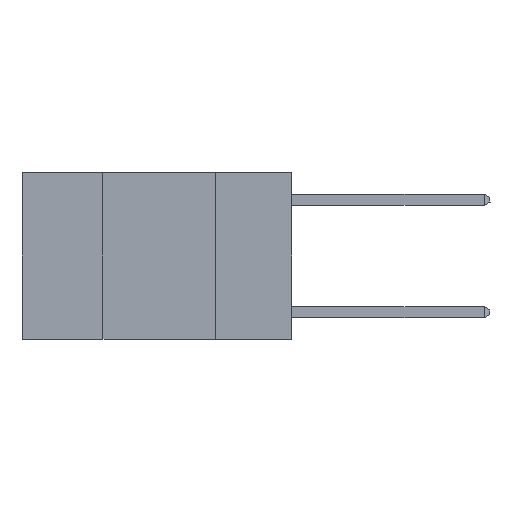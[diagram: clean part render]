
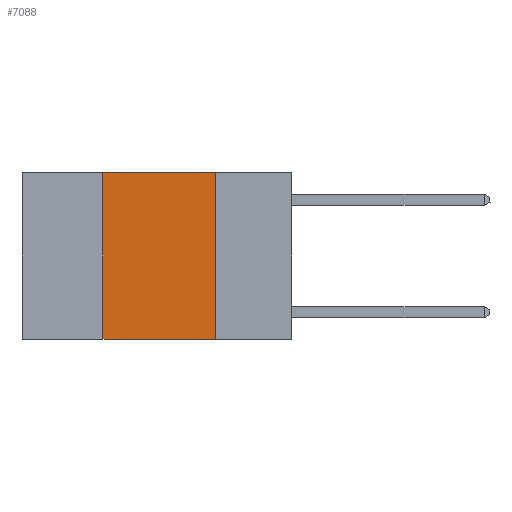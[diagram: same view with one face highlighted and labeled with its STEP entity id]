
A CAD part, left-side view. The second image highlights one B-rep face of the part: STEP entity #7088.
In plain terms, the highlighted planar face has unit normal (-1, 0, 0).
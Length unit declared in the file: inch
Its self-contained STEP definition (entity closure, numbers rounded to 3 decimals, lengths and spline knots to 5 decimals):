
#65 = CARTESIAN_POINT ( 'NONE',  ( 0., 0.6, 0. ) ) ;
#1277 = DIRECTION ( 'NONE',  ( 0., -1., 0. ) ) ;
#1431 = CARTESIAN_POINT ( 'NONE',  ( 0., 0.6, 0. ) ) ;
#1704 = LINE ( 'NONE', #65, #8877 ) ;
#2917 = DIRECTION ( 'NONE',  ( 0., 0., -1. ) ) ;
#5926 = CARTESIAN_POINT ( 'NONE',  ( 0., 0.42, -0.37 ) ) ;
#6629 = CARTESIAN_POINT ( 'NONE',  ( 0., 0.17, 0. ) ) ;
#7088 = ADVANCED_FACE ( 'NONE', ( #14624 ), #8603, .F. ) ;
#7216 = DIRECTION ( 'NONE',  ( 0., 0., 1. ) ) ;
#7532 = LINE ( 'NONE', #8627, #13760 ) ;
#8603 = PLANE ( 'NONE',  #8641 ) ;
#8627 = CARTESIAN_POINT ( 'NONE',  ( 0., 0.42, 0. ) ) ;
#8641 = AXIS2_PLACEMENT_3D ( 'NONE', #1431, #11444, #2917 ) ;
#8877 = VECTOR ( 'NONE', #17125, 39.37008 ) ;
#9831 = VERTEX_POINT ( 'NONE', #17986 ) ;
#9902 = LINE ( 'NONE', #16885, #10822 ) ;
#10078 = EDGE_CURVE ( 'NONE', #9831, #17822, #1704, .T. ) ;
#10723 = EDGE_CURVE ( 'NONE', #16892, #9831, #7532, .T. ) ;
#10822 = VECTOR ( 'NONE', #1277, 39.37008 ) ;
#11444 = DIRECTION ( 'NONE',  ( 1., 0., 0. ) ) ;
#11668 = EDGE_CURVE ( 'NONE', #16892, #16803, #9902, .T. ) ;
#13602 = EDGE_CURVE ( 'NONE', #17822, #16803, #17552, .T. ) ;
#13760 = VECTOR ( 'NONE', #7216, 39.37008 ) ;
#13881 = VECTOR ( 'NONE', #16461, 39.37008 ) ;
#14390 = ORIENTED_EDGE ( 'NONE', *, *, #13602, .F. ) ;
#14624 = FACE_OUTER_BOUND ( 'NONE', #16353, .T. ) ;
#15606 = CARTESIAN_POINT ( 'NONE',  ( 0., 0.17, -0.37 ) ) ;
#15676 = ORIENTED_EDGE ( 'NONE', *, *, #10078, .F. ) ;
#16070 = CARTESIAN_POINT ( 'NONE',  ( 0., 0.17, 0. ) ) ;
#16353 = EDGE_LOOP ( 'NONE', ( #14390, #15676, #16742, #17828 ) ) ;
#16461 = DIRECTION ( 'NONE',  ( 0., 0., -1. ) ) ;
#16742 = ORIENTED_EDGE ( 'NONE', *, *, #10723, .F. ) ;
#16803 = VERTEX_POINT ( 'NONE', #15606 ) ;
#16885 = CARTESIAN_POINT ( 'NONE',  ( 0., 0.6, -0.37 ) ) ;
#16892 = VERTEX_POINT ( 'NONE', #5926 ) ;
#17125 = DIRECTION ( 'NONE',  ( 0., -1., 0. ) ) ;
#17552 = LINE ( 'NONE', #6629, #13881 ) ;
#17822 = VERTEX_POINT ( 'NONE', #16070 ) ;
#17828 = ORIENTED_EDGE ( 'NONE', *, *, #11668, .T. ) ;
#17986 = CARTESIAN_POINT ( 'NONE',  ( 0., 0.42, 0. ) ) ;
